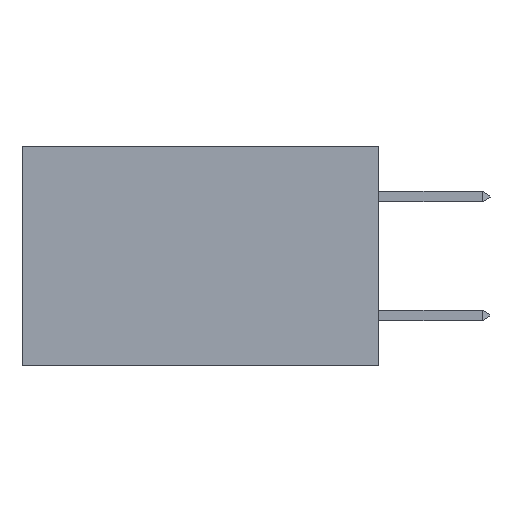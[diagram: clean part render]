
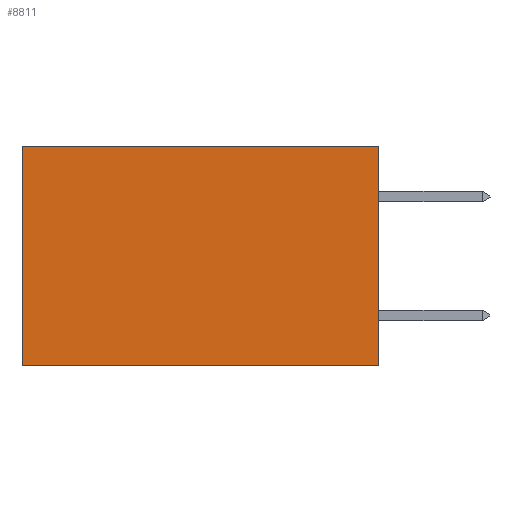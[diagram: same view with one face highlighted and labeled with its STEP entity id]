
A CAD part, left-side view. The second image highlights one B-rep face of the part: STEP entity #8811.
In plain terms, the highlighted planar face has unit normal (-1, 0, 0).
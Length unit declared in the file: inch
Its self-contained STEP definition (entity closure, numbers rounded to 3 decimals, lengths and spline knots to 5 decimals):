
#533 = CARTESIAN_POINT ( 'NONE',  ( 0.298, 0., -0.37 ) ) ;
#571 = CARTESIAN_POINT ( 'NONE',  ( 0.298, 0.6, 0. ) ) ;
#628 = CARTESIAN_POINT ( 'NONE',  ( 0.298, 0., 0. ) ) ;
#1339 = EDGE_CURVE ( 'NONE', #6697, #18755, #9492, .T. ) ;
#3538 = EDGE_CURVE ( 'NONE', #18755, #6341, #8462, .T. ) ;
#4271 = VECTOR ( 'NONE', #8455, 39.37008 ) ;
#5504 = CARTESIAN_POINT ( 'NONE',  ( 0.298, 0.6, 0. ) ) ;
#5531 = FACE_OUTER_BOUND ( 'NONE', #16817, .T. ) ;
#6341 = VERTEX_POINT ( 'NONE', #7587 ) ;
#6463 = EDGE_CURVE ( 'NONE', #16006, #6341, #8129, .T. ) ;
#6697 = VERTEX_POINT ( 'NONE', #10940 ) ;
#7327 = ORIENTED_EDGE ( 'NONE', *, *, #1339, .F. ) ;
#7587 = CARTESIAN_POINT ( 'NONE',  ( 0.298, 0.6, -0.37 ) ) ;
#7622 = AXIS2_PLACEMENT_3D ( 'NONE', #9295, #15283, #16725 ) ;
#7847 = PLANE ( 'NONE',  #7622 ) ;
#7874 = DIRECTION ( 'NONE',  ( 0., 1., 0. ) ) ;
#8129 = LINE ( 'NONE', #571, #15662 ) ;
#8455 = DIRECTION ( 'NONE',  ( 0., 1., 0. ) ) ;
#8462 = LINE ( 'NONE', #11021, #4271 ) ;
#8811 = ADVANCED_FACE ( 'NONE', ( #5531 ), #7847, .F. ) ;
#9295 = CARTESIAN_POINT ( 'NONE',  ( 0.298, 0., 0. ) ) ;
#9418 = DIRECTION ( 'NONE',  ( 0., 0., -1. ) ) ;
#9492 = LINE ( 'NONE', #628, #18931 ) ;
#9562 = CARTESIAN_POINT ( 'NONE',  ( 0.298, 0., 0. ) ) ;
#9563 = VECTOR ( 'NONE', #7874, 39.37008 ) ;
#10940 = CARTESIAN_POINT ( 'NONE',  ( 0.298, 0., 0. ) ) ;
#11021 = CARTESIAN_POINT ( 'NONE',  ( 0.298, 0., -0.37 ) ) ;
#13794 = ORIENTED_EDGE ( 'NONE', *, *, #18467, .T. ) ;
#14708 = ORIENTED_EDGE ( 'NONE', *, *, #3538, .F. ) ;
#15283 = DIRECTION ( 'NONE',  ( 1., 0., 0. ) ) ;
#15520 = DIRECTION ( 'NONE',  ( 0., 0., -1. ) ) ;
#15662 = VECTOR ( 'NONE', #9418, 39.37008 ) ;
#16006 = VERTEX_POINT ( 'NONE', #5504 ) ;
#16725 = DIRECTION ( 'NONE',  ( 0., 0., -1. ) ) ;
#16817 = EDGE_LOOP ( 'NONE', ( #17705, #14708, #7327, #13794 ) ) ;
#17705 = ORIENTED_EDGE ( 'NONE', *, *, #6463, .T. ) ;
#17846 = LINE ( 'NONE', #9562, #9563 ) ;
#18467 = EDGE_CURVE ( 'NONE', #6697, #16006, #17846, .T. ) ;
#18755 = VERTEX_POINT ( 'NONE', #533 ) ;
#18931 = VECTOR ( 'NONE', #15520, 39.37008 ) ;
